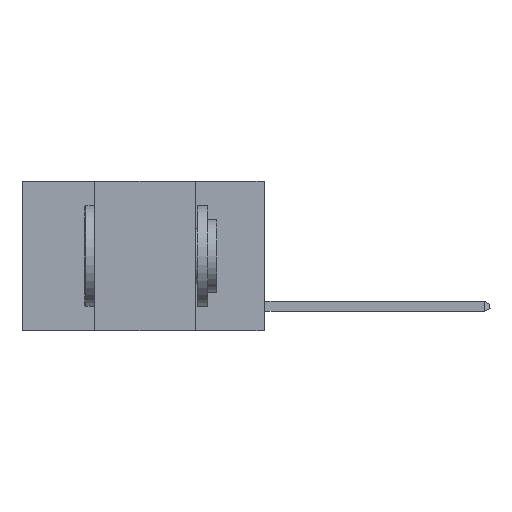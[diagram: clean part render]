
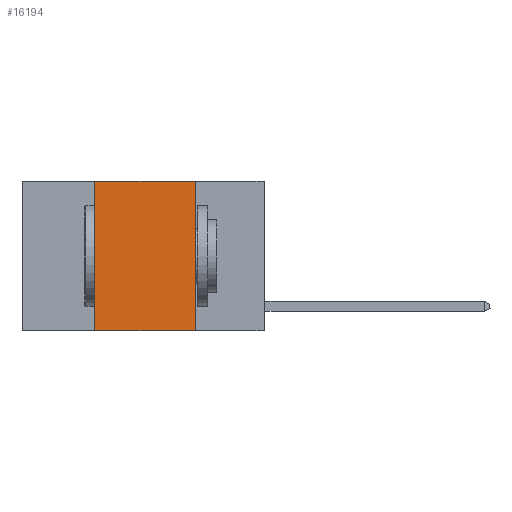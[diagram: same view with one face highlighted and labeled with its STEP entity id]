
A CAD part, left-side view. The second image highlights one B-rep face of the part: STEP entity #16194.
In plain terms, the highlighted planar face has unit normal (-1, 0, 0).
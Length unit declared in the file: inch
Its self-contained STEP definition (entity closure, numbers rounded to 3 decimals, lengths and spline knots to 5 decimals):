
#171 = LINE ( 'NONE', #13830, #17041 ) ;
#767 = ORIENTED_EDGE ( 'NONE', *, *, #5197, .F. ) ;
#1269 = DIRECTION ( 'NONE',  ( 0., -1., 0. ) ) ;
#1531 = VECTOR ( 'NONE', #3601, 39.37008 ) ;
#2034 = LINE ( 'NONE', #13270, #1531 ) ;
#2778 = LINE ( 'NONE', #18354, #15238 ) ;
#3000 = CARTESIAN_POINT ( 'NONE',  ( 0., 0.6, 0. ) ) ;
#3601 = DIRECTION ( 'NONE',  ( 0., 0., 1. ) ) ;
#4117 = AXIS2_PLACEMENT_3D ( 'NONE', #14626, #6504, #17898 ) ;
#4123 = CARTESIAN_POINT ( 'NONE',  ( 0., 0.17, 0. ) ) ;
#5197 = EDGE_CURVE ( 'NONE', #13232, #7075, #20955, .T. ) ;
#5674 = DIRECTION ( 'NONE',  ( 0., -1., 0. ) ) ;
#6504 = DIRECTION ( 'NONE',  ( 1., 0., 0. ) ) ;
#6625 = VERTEX_POINT ( 'NONE', #19400 ) ;
#7075 = VERTEX_POINT ( 'NONE', #4123 ) ;
#8026 = EDGE_CURVE ( 'NONE', #17512, #13232, #2034, .T. ) ;
#8564 = VECTOR ( 'NONE', #1269, 39.37008 ) ;
#9474 = ORIENTED_EDGE ( 'NONE', *, *, #8026, .F. ) ;
#9989 = CARTESIAN_POINT ( 'NONE',  ( 0., 0.42, 0. ) ) ;
#10259 = DIRECTION ( 'NONE',  ( 0., 0., -1. ) ) ;
#11440 = CARTESIAN_POINT ( 'NONE',  ( 0., 0.42, -0.37 ) ) ;
#11965 = EDGE_CURVE ( 'NONE', #7075, #6625, #2778, .T. ) ;
#12089 = EDGE_CURVE ( 'NONE', #17512, #6625, #171, .T. ) ;
#12975 = PLANE ( 'NONE',  #4117 ) ;
#13232 = VERTEX_POINT ( 'NONE', #9989 ) ;
#13270 = CARTESIAN_POINT ( 'NONE',  ( 0., 0.42, 0. ) ) ;
#13830 = CARTESIAN_POINT ( 'NONE',  ( 0., 0.6, -0.37 ) ) ;
#14294 = ORIENTED_EDGE ( 'NONE', *, *, #12089, .T. ) ;
#14626 = CARTESIAN_POINT ( 'NONE',  ( 0., 0.6, 0. ) ) ;
#15238 = VECTOR ( 'NONE', #10259, 39.37008 ) ;
#16194 = ADVANCED_FACE ( 'NONE', ( #16258 ), #12975, .F. ) ;
#16258 = FACE_OUTER_BOUND ( 'NONE', #17957, .T. ) ;
#17041 = VECTOR ( 'NONE', #5674, 39.37008 ) ;
#17512 = VERTEX_POINT ( 'NONE', #11440 ) ;
#17611 = ORIENTED_EDGE ( 'NONE', *, *, #11965, .F. ) ;
#17898 = DIRECTION ( 'NONE',  ( 0., 0., -1. ) ) ;
#17957 = EDGE_LOOP ( 'NONE', ( #17611, #767, #9474, #14294 ) ) ;
#18354 = CARTESIAN_POINT ( 'NONE',  ( 0., 0.17, 0. ) ) ;
#19400 = CARTESIAN_POINT ( 'NONE',  ( 0., 0.17, -0.37 ) ) ;
#20955 = LINE ( 'NONE', #3000, #8564 ) ;
